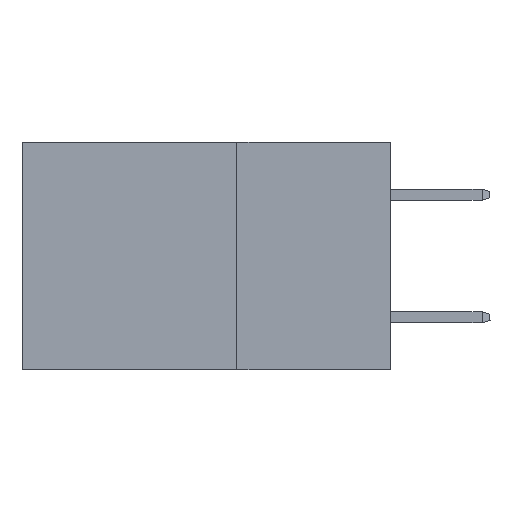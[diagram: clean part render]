
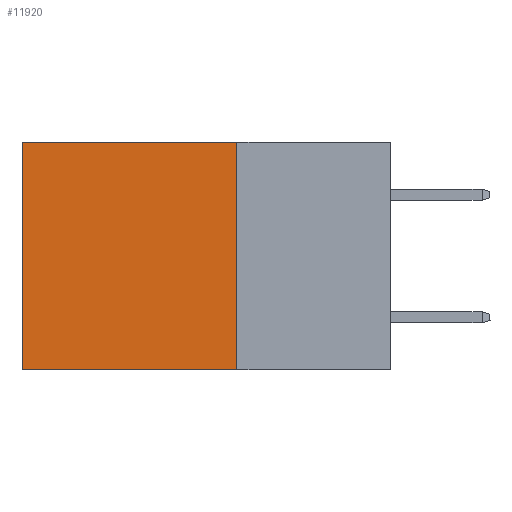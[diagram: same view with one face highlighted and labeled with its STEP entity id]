
A CAD part, left-side view. The second image highlights one B-rep face of the part: STEP entity #11920.
In plain terms, the highlighted planar face has unit normal (-1, 0, 0).
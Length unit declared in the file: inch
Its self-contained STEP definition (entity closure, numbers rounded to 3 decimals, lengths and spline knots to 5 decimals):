
#705 = LINE ( 'NONE', #31145, #29872 ) ;
#838 = DIRECTION ( 'NONE',  ( 0., 1., 0. ) ) ;
#4011 = CARTESIAN_POINT ( 'NONE',  ( 0.2875, 0.25, 0. ) ) ;
#5225 = LINE ( 'NONE', #4011, #39273 ) ;
#6133 = EDGE_CURVE ( 'NONE', #15298, #21224, #29858, .T. ) ;
#7524 = PLANE ( 'NONE',  #30060 ) ;
#9522 = ORIENTED_EDGE ( 'NONE', *, *, #34158, .T. ) ;
#10052 = EDGE_CURVE ( 'NONE', #19494, #21224, #34360, .T. ) ;
#11920 = ADVANCED_FACE ( 'NONE', ( #14221 ), #7524, .F. ) ;
#13087 = CARTESIAN_POINT ( 'NONE',  ( 0.2875, 0.25, -0.37 ) ) ;
#14221 = FACE_OUTER_BOUND ( 'NONE', #27469, .T. ) ;
#15298 = VERTEX_POINT ( 'NONE', #13087 ) ;
#17104 = ORIENTED_EDGE ( 'NONE', *, *, #36462, .F. ) ;
#17210 = DIRECTION ( 'NONE',  ( 0., 0., -1. ) ) ;
#18049 = ORIENTED_EDGE ( 'NONE', *, *, #6133, .F. ) ;
#18524 = CARTESIAN_POINT ( 'NONE',  ( 0.2875, 0.25, 0. ) ) ;
#19494 = VERTEX_POINT ( 'NONE', #36834 ) ;
#21224 = VERTEX_POINT ( 'NONE', #38723 ) ;
#21473 = CARTESIAN_POINT ( 'NONE',  ( 0.2875, 0.25, -0.37 ) ) ;
#21783 = CARTESIAN_POINT ( 'NONE',  ( 0.2875, 0.6, 0. ) ) ;
#22002 = DIRECTION ( 'NONE',  ( 0., 0., -1. ) ) ;
#24877 = VERTEX_POINT ( 'NONE', #38231 ) ;
#26588 = VECTOR ( 'NONE', #28312, 39.37008 ) ;
#27469 = EDGE_LOOP ( 'NONE', ( #38822, #18049, #17104, #9522 ) ) ;
#27770 = DIRECTION ( 'NONE',  ( 1., 0., 0. ) ) ;
#27826 = VECTOR ( 'NONE', #43558, 39.37008 ) ;
#28312 = DIRECTION ( 'NONE',  ( 0., 1., 0. ) ) ;
#29858 = LINE ( 'NONE', #21473, #26588 ) ;
#29872 = VECTOR ( 'NONE', #17210, 39.37008 ) ;
#30060 = AXIS2_PLACEMENT_3D ( 'NONE', #18524, #27770, #22002 ) ;
#31145 = CARTESIAN_POINT ( 'NONE',  ( 0.2875, 0.25, 0. ) ) ;
#34158 = EDGE_CURVE ( 'NONE', #24877, #19494, #5225, .T. ) ;
#34360 = LINE ( 'NONE', #21783, #27826 ) ;
#36462 = EDGE_CURVE ( 'NONE', #24877, #15298, #705, .T. ) ;
#36834 = CARTESIAN_POINT ( 'NONE',  ( 0.2875, 0.6, 0. ) ) ;
#38231 = CARTESIAN_POINT ( 'NONE',  ( 0.2875, 0.25, 0. ) ) ;
#38723 = CARTESIAN_POINT ( 'NONE',  ( 0.2875, 0.6, -0.37 ) ) ;
#38822 = ORIENTED_EDGE ( 'NONE', *, *, #10052, .T. ) ;
#39273 = VECTOR ( 'NONE', #838, 39.37008 ) ;
#43558 = DIRECTION ( 'NONE',  ( 0., 0., -1. ) ) ;
